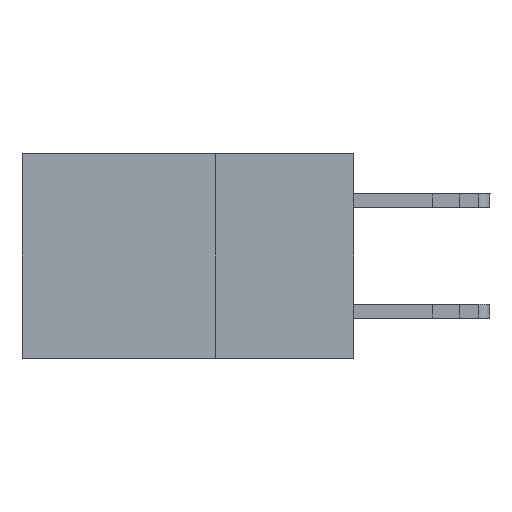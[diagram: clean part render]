
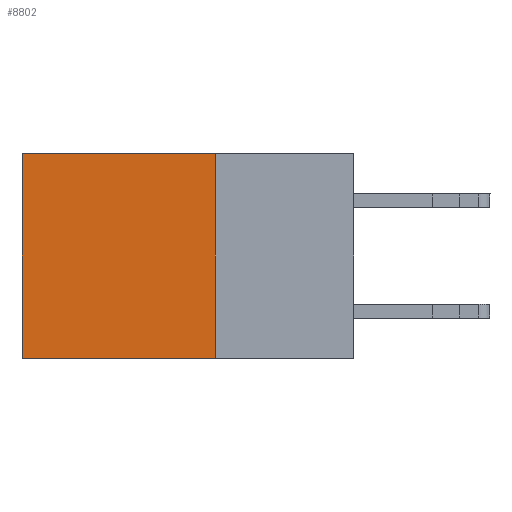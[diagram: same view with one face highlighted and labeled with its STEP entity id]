
A CAD part, left-side view. The second image highlights one B-rep face of the part: STEP entity #8802.
In plain terms, the highlighted planar face has unit normal (-1, 0, 0).
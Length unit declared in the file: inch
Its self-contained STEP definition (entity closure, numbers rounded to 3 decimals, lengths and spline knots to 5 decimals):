
#838 = DIRECTION ( 'NONE',  ( 0., 0., -1. ) ) ;
#1057 = PLANE ( 'NONE',  #4021 ) ;
#1082 = FACE_OUTER_BOUND ( 'NONE', #2339, .T. ) ;
#1506 = VERTEX_POINT ( 'NONE', #16620 ) ;
#2339 = EDGE_LOOP ( 'NONE', ( #7026, #11355, #8405, #19148 ) ) ;
#2479 = EDGE_CURVE ( 'NONE', #20395, #19266, #8016, .T. ) ;
#2837 = DIRECTION ( 'NONE',  ( 1., 0., 0. ) ) ;
#3807 = LINE ( 'NONE', #15650, #15817 ) ;
#4021 = AXIS2_PLACEMENT_3D ( 'NONE', #11141, #2837, #14335 ) ;
#4104 = VECTOR ( 'NONE', #15500, 39.37008 ) ;
#5798 = CARTESIAN_POINT ( 'NONE',  ( 0.2875, 0.25, -0.37 ) ) ;
#6544 = VERTEX_POINT ( 'NONE', #18550 ) ;
#7026 = ORIENTED_EDGE ( 'NONE', *, *, #2479, .T. ) ;
#8016 = LINE ( 'NONE', #21056, #15540 ) ;
#8320 = DIRECTION ( 'NONE',  ( 0., 0., -1. ) ) ;
#8405 = ORIENTED_EDGE ( 'NONE', *, *, #8691, .F. ) ;
#8691 = EDGE_CURVE ( 'NONE', #6544, #1506, #3807, .T. ) ;
#8802 = ADVANCED_FACE ( 'NONE', ( #1082 ), #1057, .F. ) ;
#8855 = VECTOR ( 'NONE', #19632, 39.37008 ) ;
#9144 = CARTESIAN_POINT ( 'NONE',  ( 0.2875, 0.6, 0. ) ) ;
#9886 = LINE ( 'NONE', #13319, #8855 ) ;
#11141 = CARTESIAN_POINT ( 'NONE',  ( 0.2875, 0.25, 0. ) ) ;
#11355 = ORIENTED_EDGE ( 'NONE', *, *, #20190, .F. ) ;
#11646 = CARTESIAN_POINT ( 'NONE',  ( 0.2875, 0.6, -0.37 ) ) ;
#13319 = CARTESIAN_POINT ( 'NONE',  ( 0.2875, 0.25, 0. ) ) ;
#13374 = LINE ( 'NONE', #5798, #4104 ) ;
#13827 = EDGE_CURVE ( 'NONE', #6544, #20395, #9886, .T. ) ;
#14335 = DIRECTION ( 'NONE',  ( 0., 0., -1. ) ) ;
#15500 = DIRECTION ( 'NONE',  ( 0., 1., 0. ) ) ;
#15540 = VECTOR ( 'NONE', #8320, 39.37008 ) ;
#15650 = CARTESIAN_POINT ( 'NONE',  ( 0.2875, 0.25, 0. ) ) ;
#15817 = VECTOR ( 'NONE', #838, 39.37008 ) ;
#16620 = CARTESIAN_POINT ( 'NONE',  ( 0.2875, 0.25, -0.37 ) ) ;
#18550 = CARTESIAN_POINT ( 'NONE',  ( 0.2875, 0.25, 0. ) ) ;
#19148 = ORIENTED_EDGE ( 'NONE', *, *, #13827, .T. ) ;
#19266 = VERTEX_POINT ( 'NONE', #11646 ) ;
#19632 = DIRECTION ( 'NONE',  ( 0., 1., 0. ) ) ;
#20190 = EDGE_CURVE ( 'NONE', #1506, #19266, #13374, .T. ) ;
#20395 = VERTEX_POINT ( 'NONE', #9144 ) ;
#21056 = CARTESIAN_POINT ( 'NONE',  ( 0.2875, 0.6, 0. ) ) ;
